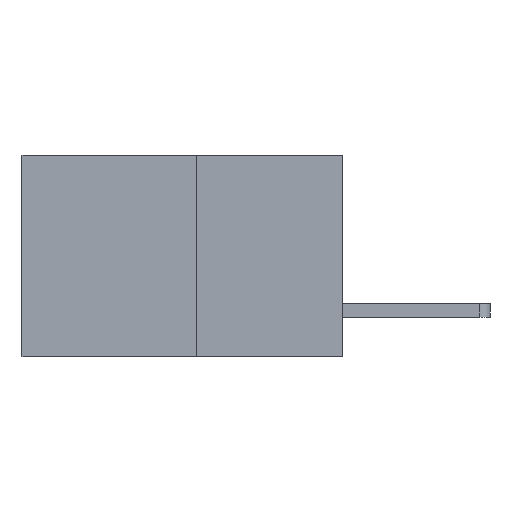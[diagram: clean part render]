
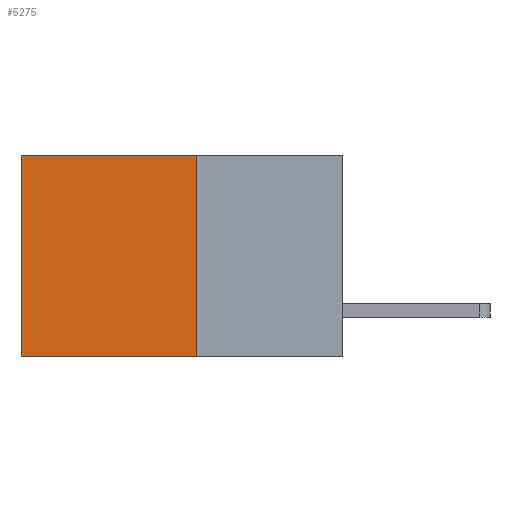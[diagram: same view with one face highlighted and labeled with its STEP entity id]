
A CAD part, left-side view. The second image highlights one B-rep face of the part: STEP entity #5275.
In plain terms, the highlighted planar face has unit normal (-1, 0, 0).
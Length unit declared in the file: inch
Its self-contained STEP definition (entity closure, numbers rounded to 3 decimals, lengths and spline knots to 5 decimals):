
#42 = LINE ( 'NONE', #6095, #4572 ) ;
#615 = DIRECTION ( 'NONE',  ( 0., 0., -1. ) ) ;
#918 = CARTESIAN_POINT ( 'NONE',  ( 0.277, 0.27, -0.37 ) ) ;
#989 = ORIENTED_EDGE ( 'NONE', *, *, #7094, .T. ) ;
#1271 = EDGE_CURVE ( 'NONE', #3389, #1609, #5994, .T. ) ;
#1609 = VERTEX_POINT ( 'NONE', #4158 ) ;
#1690 = LINE ( 'NONE', #3211, #4762 ) ;
#2061 = DIRECTION ( 'NONE',  ( 1., 0., 0. ) ) ;
#2684 = DIRECTION ( 'NONE',  ( 0., 0., -1. ) ) ;
#2805 = LINE ( 'NONE', #3449, #6119 ) ;
#3144 = CARTESIAN_POINT ( 'NONE',  ( 0.277, 0.27, 0. ) ) ;
#3211 = CARTESIAN_POINT ( 'NONE',  ( 0.277, 0.59, -0.37 ) ) ;
#3242 = PLANE ( 'NONE',  #4635 ) ;
#3389 = VERTEX_POINT ( 'NONE', #3144 ) ;
#3449 = CARTESIAN_POINT ( 'NONE',  ( 0.277, 0.27, 0. ) ) ;
#3583 = VERTEX_POINT ( 'NONE', #4486 ) ;
#4158 = CARTESIAN_POINT ( 'NONE',  ( 0.277, 0.27, -0.37 ) ) ;
#4195 = ORIENTED_EDGE ( 'NONE', *, *, #1271, .F. ) ;
#4273 = VERTEX_POINT ( 'NONE', #6969 ) ;
#4486 = CARTESIAN_POINT ( 'NONE',  ( 0.277, 0.59, -0.37 ) ) ;
#4572 = VECTOR ( 'NONE', #6667, 39.37008 ) ;
#4635 = AXIS2_PLACEMENT_3D ( 'NONE', #5614, #2061, #6182 ) ;
#4762 = VECTOR ( 'NONE', #615, 39.37008 ) ;
#5275 = ADVANCED_FACE ( 'NONE', ( #5788 ), #3242, .F. ) ;
#5614 = CARTESIAN_POINT ( 'NONE',  ( 0.277, 0.27, -0.37 ) ) ;
#5788 = FACE_OUTER_BOUND ( 'NONE', #7359, .T. ) ;
#5994 = LINE ( 'NONE', #918, #7357 ) ;
#6039 = ORIENTED_EDGE ( 'NONE', *, *, #6101, .F. ) ;
#6095 = CARTESIAN_POINT ( 'NONE',  ( 0.277, 0.27, -0.37 ) ) ;
#6101 = EDGE_CURVE ( 'NONE', #1609, #3583, #42, .T. ) ;
#6119 = VECTOR ( 'NONE', #7560, 39.37008 ) ;
#6182 = DIRECTION ( 'NONE',  ( 0., 0., -1. ) ) ;
#6603 = ORIENTED_EDGE ( 'NONE', *, *, #6973, .T. ) ;
#6667 = DIRECTION ( 'NONE',  ( 0., 1., 0. ) ) ;
#6969 = CARTESIAN_POINT ( 'NONE',  ( 0.277, 0.59, 0. ) ) ;
#6973 = EDGE_CURVE ( 'NONE', #3389, #4273, #2805, .T. ) ;
#7094 = EDGE_CURVE ( 'NONE', #4273, #3583, #1690, .T. ) ;
#7357 = VECTOR ( 'NONE', #2684, 39.37008 ) ;
#7359 = EDGE_LOOP ( 'NONE', ( #989, #6039, #4195, #6603 ) ) ;
#7560 = DIRECTION ( 'NONE',  ( 0., 1., 0. ) ) ;
